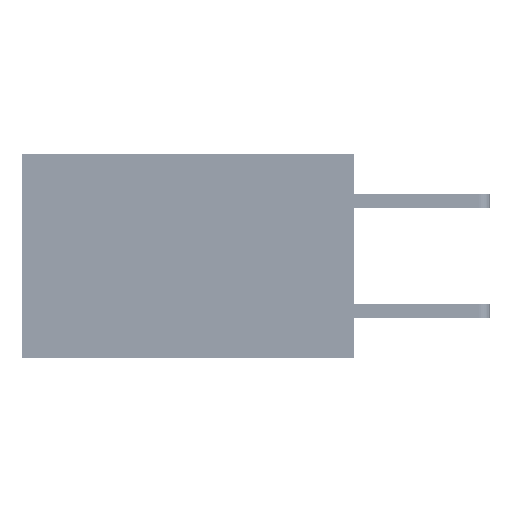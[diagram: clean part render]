
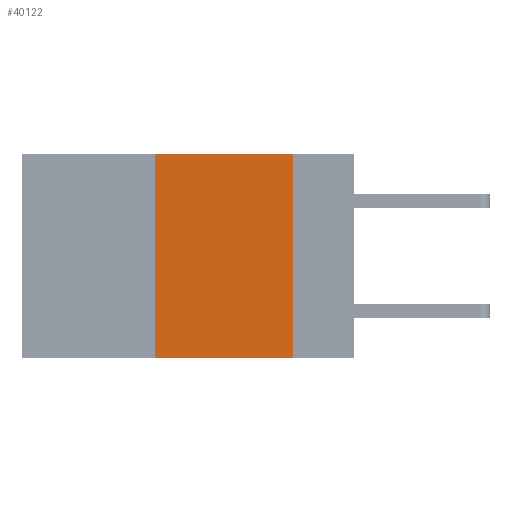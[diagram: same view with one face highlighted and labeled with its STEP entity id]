
A CAD part, left-side view. The second image highlights one B-rep face of the part: STEP entity #40122.
In plain terms, the highlighted planar face has unit normal (-1, 0, 0).
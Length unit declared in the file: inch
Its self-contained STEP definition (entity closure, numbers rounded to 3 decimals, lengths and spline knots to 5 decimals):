
#2840 = EDGE_CURVE ( 'NONE', #12045, #4657, #4501, .T. ) ;
#4501 = LINE ( 'NONE', #32239, #28781 ) ;
#4657 = VERTEX_POINT ( 'NONE', #40733 ) ;
#5940 = AXIS2_PLACEMENT_3D ( 'NONE', #12981, #35070, #16169 ) ;
#6144 = ORIENTED_EDGE ( 'NONE', *, *, #39761, .T. ) ;
#6584 = LINE ( 'NONE', #34800, #13026 ) ;
#8484 = EDGE_CURVE ( 'NONE', #4657, #37369, #31257, .T. ) ;
#9649 = EDGE_LOOP ( 'NONE', ( #22492, #25481, #36755, #6144 ) ) ;
#11224 = CARTESIAN_POINT ( 'NONE',  ( 0., 0.6, -0.37 ) ) ;
#12045 = VERTEX_POINT ( 'NONE', #32910 ) ;
#12713 = DIRECTION ( 'NONE',  ( 0., 0., 1. ) ) ;
#12981 = CARTESIAN_POINT ( 'NONE',  ( 0., 0.6, 0. ) ) ;
#13026 = VECTOR ( 'NONE', #12713, 39.37008 ) ;
#13783 = FACE_OUTER_BOUND ( 'NONE', #9649, .T. ) ;
#16026 = PLANE ( 'NONE',  #5940 ) ;
#16169 = DIRECTION ( 'NONE',  ( 0., 0., -1. ) ) ;
#18509 = VERTEX_POINT ( 'NONE', #40318 ) ;
#19384 = CARTESIAN_POINT ( 'NONE',  ( 0., 0.11, -0.37 ) ) ;
#20982 = CARTESIAN_POINT ( 'NONE',  ( 0., 0.11, 0. ) ) ;
#22492 = ORIENTED_EDGE ( 'NONE', *, *, #8484, .F. ) ;
#22857 = VECTOR ( 'NONE', #30530, 39.37008 ) ;
#25481 = ORIENTED_EDGE ( 'NONE', *, *, #2840, .F. ) ;
#25932 = VECTOR ( 'NONE', #39544, 39.37008 ) ;
#28781 = VECTOR ( 'NONE', #35381, 39.37008 ) ;
#30530 = DIRECTION ( 'NONE',  ( 0., 0., -1. ) ) ;
#31257 = LINE ( 'NONE', #20982, #22857 ) ;
#32239 = CARTESIAN_POINT ( 'NONE',  ( 0., 0.6, 0. ) ) ;
#32910 = CARTESIAN_POINT ( 'NONE',  ( 0., 0.36, 0. ) ) ;
#34300 = LINE ( 'NONE', #11224, #25932 ) ;
#34800 = CARTESIAN_POINT ( 'NONE',  ( 0., 0.36, 0. ) ) ;
#35070 = DIRECTION ( 'NONE',  ( 1., 0., 0. ) ) ;
#35381 = DIRECTION ( 'NONE',  ( 0., -1., 0. ) ) ;
#36755 = ORIENTED_EDGE ( 'NONE', *, *, #40087, .F. ) ;
#37369 = VERTEX_POINT ( 'NONE', #19384 ) ;
#39544 = DIRECTION ( 'NONE',  ( 0., -1., 0. ) ) ;
#39761 = EDGE_CURVE ( 'NONE', #18509, #37369, #34300, .T. ) ;
#40087 = EDGE_CURVE ( 'NONE', #18509, #12045, #6584, .T. ) ;
#40122 = ADVANCED_FACE ( 'NONE', ( #13783 ), #16026, .F. ) ;
#40318 = CARTESIAN_POINT ( 'NONE',  ( 0., 0.36, -0.37 ) ) ;
#40733 = CARTESIAN_POINT ( 'NONE',  ( 0., 0.11, 0. ) ) ;
